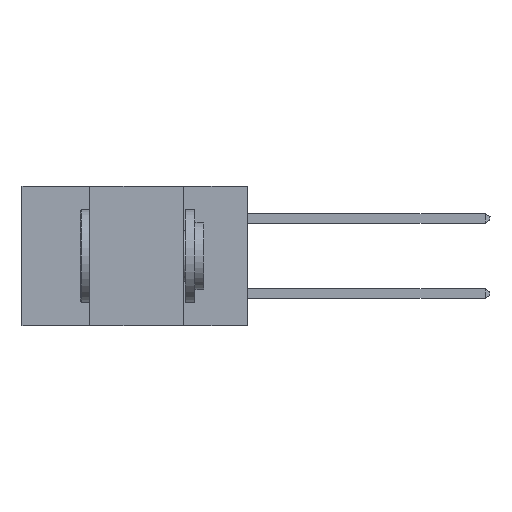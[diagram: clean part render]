
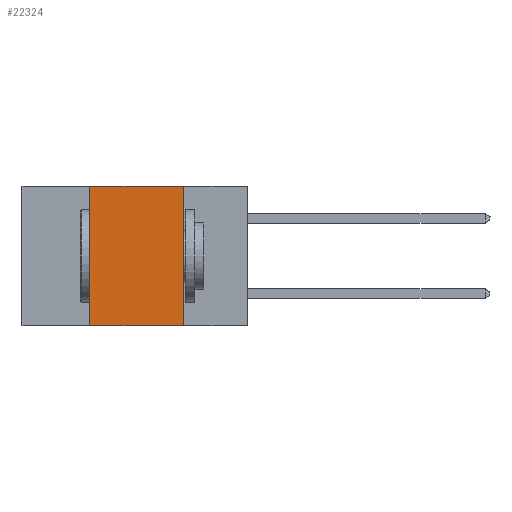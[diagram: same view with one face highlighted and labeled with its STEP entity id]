
A CAD part, left-side view. The second image highlights one B-rep face of the part: STEP entity #22324.
In plain terms, the highlighted planar face has unit normal (-1, 0, 0).
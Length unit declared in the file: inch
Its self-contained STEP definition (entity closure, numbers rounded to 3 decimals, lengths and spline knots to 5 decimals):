
#1177 = CARTESIAN_POINT ( 'NONE',  ( 0., 0.42, -0.37 ) ) ;
#1264 = EDGE_CURVE ( 'NONE', #23248, #13043, #18405, .T. ) ;
#2792 = DIRECTION ( 'NONE',  ( 0., 0., -1. ) ) ;
#3134 = ORIENTED_EDGE ( 'NONE', *, *, #13933, .F. ) ;
#3341 = VERTEX_POINT ( 'NONE', #19987 ) ;
#3921 = ORIENTED_EDGE ( 'NONE', *, *, #1264, .F. ) ;
#4400 = EDGE_CURVE ( 'NONE', #13043, #8401, #6762, .T. ) ;
#4534 = DIRECTION ( 'NONE',  ( 0., 0., 1. ) ) ;
#5705 = CARTESIAN_POINT ( 'NONE',  ( 0., 0.17, 0. ) ) ;
#6060 = CARTESIAN_POINT ( 'NONE',  ( 0., 0.17, 0. ) ) ;
#6114 = VECTOR ( 'NONE', #10975, 39.37008 ) ;
#6557 = LINE ( 'NONE', #6060, #25113 ) ;
#6762 = LINE ( 'NONE', #29216, #17390 ) ;
#7624 = CARTESIAN_POINT ( 'NONE',  ( 0., 0.6, 0. ) ) ;
#8120 = CARTESIAN_POINT ( 'NONE',  ( 0., 0.6, -0.37 ) ) ;
#8401 = VERTEX_POINT ( 'NONE', #5705 ) ;
#9621 = CARTESIAN_POINT ( 'NONE',  ( 0., 0.42, 0. ) ) ;
#9975 = ORIENTED_EDGE ( 'NONE', *, *, #11455, .T. ) ;
#10975 = DIRECTION ( 'NONE',  ( 0., -1., 0. ) ) ;
#11455 = EDGE_CURVE ( 'NONE', #23248, #3341, #30359, .T. ) ;
#11568 = VECTOR ( 'NONE', #4534, 39.37008 ) ;
#13043 = VERTEX_POINT ( 'NONE', #9621 ) ;
#13933 = EDGE_CURVE ( 'NONE', #8401, #3341, #6557, .T. ) ;
#16874 = DIRECTION ( 'NONE',  ( 0., -1., 0. ) ) ;
#17362 = DIRECTION ( 'NONE',  ( 1., 0., 0. ) ) ;
#17390 = VECTOR ( 'NONE', #16874, 39.37008 ) ;
#18405 = LINE ( 'NONE', #21594, #11568 ) ;
#19987 = CARTESIAN_POINT ( 'NONE',  ( 0., 0.17, -0.37 ) ) ;
#21594 = CARTESIAN_POINT ( 'NONE',  ( 0., 0.42, 0. ) ) ;
#22136 = PLANE ( 'NONE',  #27832 ) ;
#22324 = ADVANCED_FACE ( 'NONE', ( #30891 ), #22136, .F. ) ;
#23248 = VERTEX_POINT ( 'NONE', #1177 ) ;
#25113 = VECTOR ( 'NONE', #30088, 39.37008 ) ;
#27832 = AXIS2_PLACEMENT_3D ( 'NONE', #7624, #17362, #2792 ) ;
#28474 = EDGE_LOOP ( 'NONE', ( #3134, #31430, #3921, #9975 ) ) ;
#29216 = CARTESIAN_POINT ( 'NONE',  ( 0., 0.6, 0. ) ) ;
#30088 = DIRECTION ( 'NONE',  ( 0., 0., -1. ) ) ;
#30359 = LINE ( 'NONE', #8120, #6114 ) ;
#30891 = FACE_OUTER_BOUND ( 'NONE', #28474, .T. ) ;
#31430 = ORIENTED_EDGE ( 'NONE', *, *, #4400, .F. ) ;
